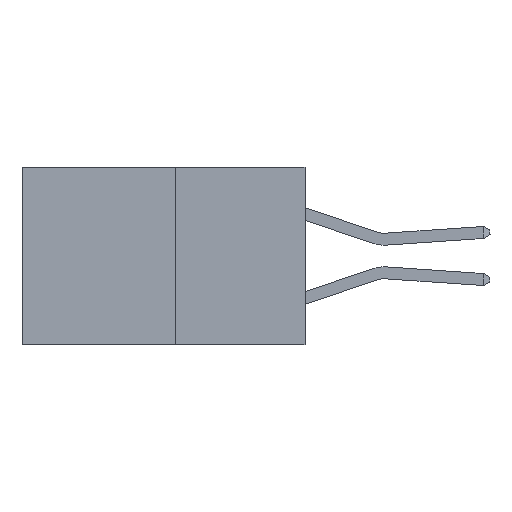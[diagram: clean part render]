
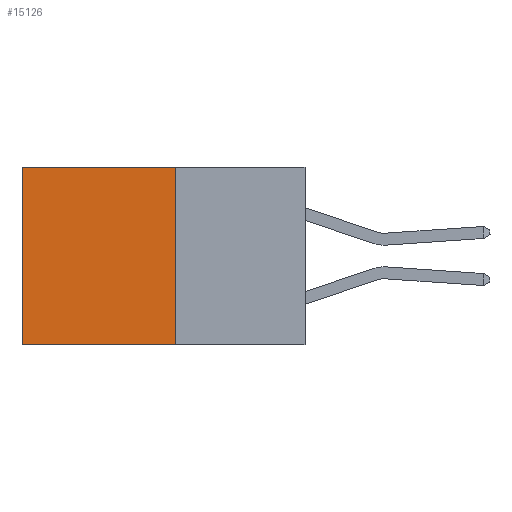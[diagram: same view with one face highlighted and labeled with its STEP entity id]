
A CAD part, left-side view. The second image highlights one B-rep face of the part: STEP entity #15126.
In plain terms, the highlighted planar face has unit normal (-1, 0, 0).
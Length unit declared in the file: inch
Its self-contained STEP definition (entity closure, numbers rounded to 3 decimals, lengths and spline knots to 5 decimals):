
#341 = DIRECTION ( 'NONE',  ( 1., 0., 0. ) ) ;
#368 = VERTEX_POINT ( 'NONE', #7891 ) ;
#494 = CARTESIAN_POINT ( 'NONE',  ( 0.277, 0.59, -0.37 ) ) ;
#833 = VERTEX_POINT ( 'NONE', #9365 ) ;
#1132 = VECTOR ( 'NONE', #14192, 39.37008 ) ;
#1690 = CARTESIAN_POINT ( 'NONE',  ( 0.277, 0.59, -0.37 ) ) ;
#2178 = DIRECTION ( 'NONE',  ( 0., 0., -1. ) ) ;
#2210 = DIRECTION ( 'NONE',  ( 0., 0., -1. ) ) ;
#3877 = VECTOR ( 'NONE', #9965, 39.37008 ) ;
#5103 = ORIENTED_EDGE ( 'NONE', *, *, #8528, .T. ) ;
#5124 = ORIENTED_EDGE ( 'NONE', *, *, #15641, .T. ) ;
#6558 = LINE ( 'NONE', #19567, #14420 ) ;
#7384 = EDGE_CURVE ( 'NONE', #833, #10809, #8785, .T. ) ;
#7891 = CARTESIAN_POINT ( 'NONE',  ( 0.277, 0.59, 0. ) ) ;
#8446 = CARTESIAN_POINT ( 'NONE',  ( 0.277, 0.27, -0.37 ) ) ;
#8497 = LINE ( 'NONE', #1690, #8988 ) ;
#8528 = EDGE_CURVE ( 'NONE', #368, #10809, #8497, .T. ) ;
#8785 = LINE ( 'NONE', #10182, #3877 ) ;
#8988 = VECTOR ( 'NONE', #2178, 39.37008 ) ;
#9103 = CARTESIAN_POINT ( 'NONE',  ( 0.277, 0.27, 0. ) ) ;
#9365 = CARTESIAN_POINT ( 'NONE',  ( 0.277, 0.27, -0.37 ) ) ;
#9965 = DIRECTION ( 'NONE',  ( 0., 1., 0. ) ) ;
#10123 = PLANE ( 'NONE',  #17111 ) ;
#10182 = CARTESIAN_POINT ( 'NONE',  ( 0.277, 0.27, -0.37 ) ) ;
#10809 = VERTEX_POINT ( 'NONE', #494 ) ;
#11665 = DIRECTION ( 'NONE',  ( 0., 0., -1. ) ) ;
#13424 = LINE ( 'NONE', #14257, #1132 ) ;
#14026 = EDGE_CURVE ( 'NONE', #20413, #833, #6558, .T. ) ;
#14192 = DIRECTION ( 'NONE',  ( 0., 1., 0. ) ) ;
#14257 = CARTESIAN_POINT ( 'NONE',  ( 0.277, 0.27, 0. ) ) ;
#14420 = VECTOR ( 'NONE', #2210, 39.37008 ) ;
#14766 = ORIENTED_EDGE ( 'NONE', *, *, #14026, .F. ) ;
#15126 = ADVANCED_FACE ( 'NONE', ( #18030 ), #10123, .F. ) ;
#15641 = EDGE_CURVE ( 'NONE', #20413, #368, #13424, .T. ) ;
#16446 = ORIENTED_EDGE ( 'NONE', *, *, #7384, .F. ) ;
#17111 = AXIS2_PLACEMENT_3D ( 'NONE', #8446, #341, #11665 ) ;
#18030 = FACE_OUTER_BOUND ( 'NONE', #19027, .T. ) ;
#19027 = EDGE_LOOP ( 'NONE', ( #5103, #16446, #14766, #5124 ) ) ;
#19567 = CARTESIAN_POINT ( 'NONE',  ( 0.277, 0.27, -0.37 ) ) ;
#20413 = VERTEX_POINT ( 'NONE', #9103 ) ;
